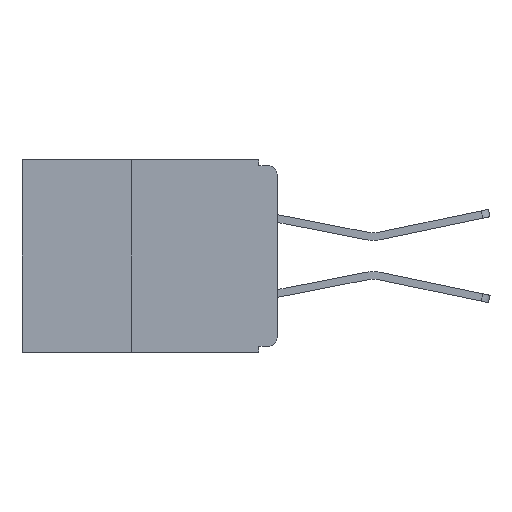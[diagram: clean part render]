
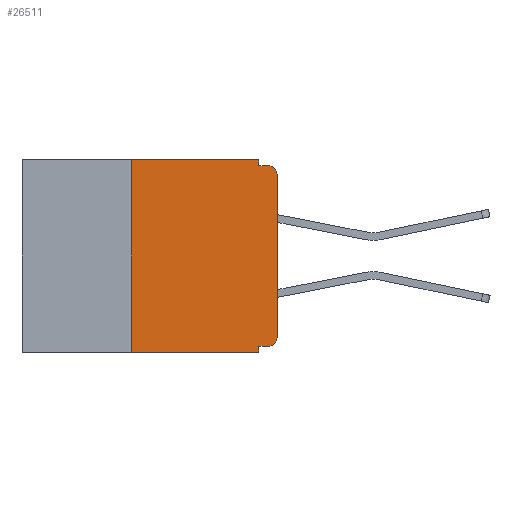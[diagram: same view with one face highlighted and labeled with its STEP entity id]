
A CAD part, left-side view. The second image highlights one B-rep face of the part: STEP entity #26511.
In plain terms, the highlighted planar face has unit normal (-1, 0, 0).
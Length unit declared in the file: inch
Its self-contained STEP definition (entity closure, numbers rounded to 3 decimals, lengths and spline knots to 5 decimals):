
#136 = LINE ( 'NONE', #570, #26260 ) ;
#244 = VECTOR ( 'NONE', #5944, 39.37008 ) ;
#346 = CARTESIAN_POINT ( 'NONE',  ( 0., 0.031, -0.01 ) ) ;
#459 = VERTEX_POINT ( 'NONE', #30499 ) ;
#570 = CARTESIAN_POINT ( 'NONE',  ( 0., 0., -0.01 ) ) ;
#907 = EDGE_CURVE ( 'NONE', #26278, #1186, #136, .T. ) ;
#1104 = CARTESIAN_POINT ( 'NONE',  ( 0., 0.25, -0.33 ) ) ;
#1152 = DIRECTION ( 'NONE',  ( 0., 1., 0. ) ) ;
#1186 = VERTEX_POINT ( 'NONE', #5646 ) ;
#1307 = DIRECTION ( 'NONE',  ( 0., -1., 0. ) ) ;
#1311 = EDGE_LOOP ( 'NONE', ( #13461, #25500, #12276, #10160, #5288, #13875, #31704, #16925, #29978, #25604 ) ) ;
#1418 = DIRECTION ( 'NONE',  ( -1., 0., 0. ) ) ;
#1780 = CARTESIAN_POINT ( 'NONE',  ( 0., 0., -0.32 ) ) ;
#1952 = AXIS2_PLACEMENT_3D ( 'NONE', #16671, #1418, #19139 ) ;
#2126 = EDGE_CURVE ( 'NONE', #24917, #28844, #25794, .T. ) ;
#3243 = CIRCLE ( 'NONE', #1952, 0.015 ) ;
#3490 = DIRECTION ( 'NONE',  ( 0., -1., 0. ) ) ;
#3757 = CARTESIAN_POINT ( 'NONE',  ( 0., 0.031, -0.32 ) ) ;
#4925 = VECTOR ( 'NONE', #1307, 39.37008 ) ;
#5288 = ORIENTED_EDGE ( 'NONE', *, *, #27656, .F. ) ;
#5646 = CARTESIAN_POINT ( 'NONE',  ( 0., 0.015, -0.01 ) ) ;
#5802 = CARTESIAN_POINT ( 'NONE',  ( 0., 0.031, 0. ) ) ;
#5944 = DIRECTION ( 'NONE',  ( 0., -1., 0. ) ) ;
#6087 = CARTESIAN_POINT ( 'NONE',  ( 0., 0.25, -0.33 ) ) ;
#6662 = LINE ( 'NONE', #6087, #31819 ) ;
#7030 = DIRECTION ( 'NONE',  ( 1., 0., 0. ) ) ;
#7639 = EDGE_CURVE ( 'NONE', #459, #11130, #19572, .T. ) ;
#7794 = VERTEX_POINT ( 'NONE', #1104 ) ;
#8540 = CARTESIAN_POINT ( 'NONE',  ( 0., 0.031, -0.33 ) ) ;
#10160 = ORIENTED_EDGE ( 'NONE', *, *, #14595, .F. ) ;
#11130 = VERTEX_POINT ( 'NONE', #30945 ) ;
#11187 = LINE ( 'NONE', #22832, #23659 ) ;
#11288 = CARTESIAN_POINT ( 'NONE',  ( 0., 0.031, 0. ) ) ;
#12028 = CARTESIAN_POINT ( 'NONE',  ( 0., 0.437, 0. ) ) ;
#12185 = VECTOR ( 'NONE', #13307, 39.37008 ) ;
#12276 = ORIENTED_EDGE ( 'NONE', *, *, #907, .F. ) ;
#12283 = VERTEX_POINT ( 'NONE', #13228 ) ;
#12698 = FACE_OUTER_BOUND ( 'NONE', #1311, .T. ) ;
#13228 = CARTESIAN_POINT ( 'NONE',  ( 0., 0.25, 0. ) ) ;
#13307 = DIRECTION ( 'NONE',  ( 0., 0., 1. ) ) ;
#13461 = ORIENTED_EDGE ( 'NONE', *, *, #7639, .T. ) ;
#13622 = EDGE_CURVE ( 'NONE', #7794, #21329, #13856, .T. ) ;
#13668 = DIRECTION ( 'NONE',  ( -1., 0., 0. ) ) ;
#13856 = LINE ( 'NONE', #23483, #244 ) ;
#13875 = ORIENTED_EDGE ( 'NONE', *, *, #32057, .F. ) ;
#14595 = EDGE_CURVE ( 'NONE', #15087, #26278, #24727, .T. ) ;
#15087 = VERTEX_POINT ( 'NONE', #5802 ) ;
#15884 = AXIS2_PLACEMENT_3D ( 'NONE', #12028, #7030, #24572 ) ;
#16671 = CARTESIAN_POINT ( 'NONE',  ( 0., 0.015, -0.305 ) ) ;
#16925 = ORIENTED_EDGE ( 'NONE', *, *, #29858, .F. ) ;
#17560 = LINE ( 'NONE', #31582, #4925 ) ;
#17849 = DIRECTION ( 'NONE',  ( 0., 0., -1. ) ) ;
#18358 = VECTOR ( 'NONE', #1152, 39.37008 ) ;
#18803 = DIRECTION ( 'NONE',  ( 0., 0., -1. ) ) ;
#19139 = DIRECTION ( 'NONE',  ( 0., 0., -1. ) ) ;
#19521 = PLANE ( 'NONE',  #15884 ) ;
#19572 = LINE ( 'NONE', #25755, #12185 ) ;
#21329 = VERTEX_POINT ( 'NONE', #8540 ) ;
#22832 = CARTESIAN_POINT ( 'NONE',  ( 0., 0.031, -0.33 ) ) ;
#23483 = CARTESIAN_POINT ( 'NONE',  ( 0., 0.437, -0.33 ) ) ;
#23659 = VECTOR ( 'NONE', #17849, 39.37008 ) ;
#23919 = VECTOR ( 'NONE', #18803, 39.37008 ) ;
#24572 = DIRECTION ( 'NONE',  ( 0., 0., -1. ) ) ;
#24727 = LINE ( 'NONE', #11288, #23919 ) ;
#24822 = CIRCLE ( 'NONE', #30036, 0.015 ) ;
#24917 = VERTEX_POINT ( 'NONE', #31365 ) ;
#24969 = EDGE_CURVE ( 'NONE', #24917, #459, #3243, .T. ) ;
#25500 = ORIENTED_EDGE ( 'NONE', *, *, #30571, .T. ) ;
#25604 = ORIENTED_EDGE ( 'NONE', *, *, #24969, .T. ) ;
#25755 = CARTESIAN_POINT ( 'NONE',  ( 0., 0., 0. ) ) ;
#25794 = LINE ( 'NONE', #1780, #18358 ) ;
#26172 = DIRECTION ( 'NONE',  ( 0., 0., 1. ) ) ;
#26260 = VECTOR ( 'NONE', #3490, 39.37008 ) ;
#26278 = VERTEX_POINT ( 'NONE', #346 ) ;
#26511 = ADVANCED_FACE ( 'NONE', ( #12698 ), #19521, .F. ) ;
#27656 = EDGE_CURVE ( 'NONE', #12283, #15087, #17560, .T. ) ;
#28680 = CARTESIAN_POINT ( 'NONE',  ( 0., 0.015, -0.025 ) ) ;
#28844 = VERTEX_POINT ( 'NONE', #3757 ) ;
#29858 = EDGE_CURVE ( 'NONE', #28844, #21329, #11187, .T. ) ;
#29978 = ORIENTED_EDGE ( 'NONE', *, *, #2126, .F. ) ;
#30036 = AXIS2_PLACEMENT_3D ( 'NONE', #28680, #13668, #31213 ) ;
#30499 = CARTESIAN_POINT ( 'NONE',  ( 0., 0., -0.305 ) ) ;
#30571 = EDGE_CURVE ( 'NONE', #11130, #1186, #24822, .T. ) ;
#30945 = CARTESIAN_POINT ( 'NONE',  ( 0., 0., -0.025 ) ) ;
#31213 = DIRECTION ( 'NONE',  ( 0., 0., -1. ) ) ;
#31365 = CARTESIAN_POINT ( 'NONE',  ( 0., 0.015, -0.32 ) ) ;
#31582 = CARTESIAN_POINT ( 'NONE',  ( 0., 0.437, 0. ) ) ;
#31704 = ORIENTED_EDGE ( 'NONE', *, *, #13622, .T. ) ;
#31819 = VECTOR ( 'NONE', #26172, 39.37008 ) ;
#32057 = EDGE_CURVE ( 'NONE', #7794, #12283, #6662, .T. ) ;
